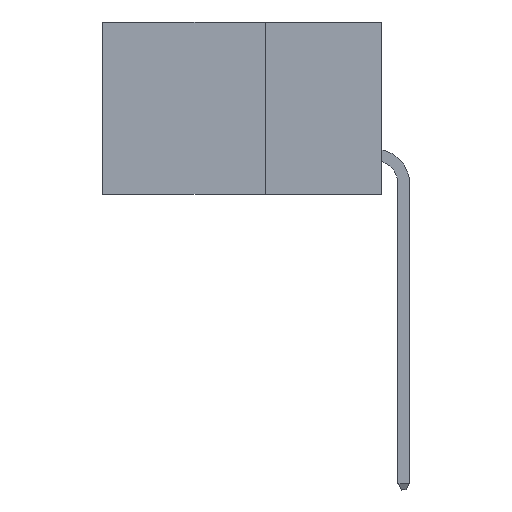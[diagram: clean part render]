
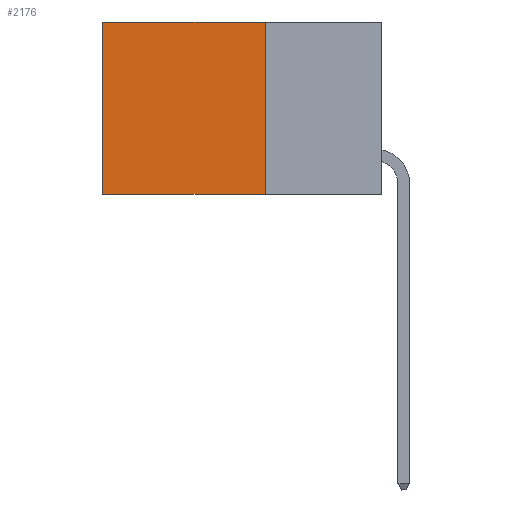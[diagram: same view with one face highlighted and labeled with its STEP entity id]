
A CAD part, left-side view. The second image highlights one B-rep face of the part: STEP entity #2176.
In plain terms, the highlighted planar face has unit normal (-1, 0, 0).
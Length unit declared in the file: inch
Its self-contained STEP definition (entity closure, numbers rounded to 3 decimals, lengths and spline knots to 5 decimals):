
#363 = CARTESIAN_POINT ( 'NONE',  ( 0.2875, 0.25, -0.37 ) ) ;
#565 = CARTESIAN_POINT ( 'NONE',  ( 0.2875, 0.6, -0.37 ) ) ;
#636 = AXIS2_PLACEMENT_3D ( 'NONE', #1433, #10157, #8273 ) ;
#751 = VECTOR ( 'NONE', #8281, 39.37008 ) ;
#756 = VERTEX_POINT ( 'NONE', #565 ) ;
#850 = ORIENTED_EDGE ( 'NONE', *, *, #8083, .T. ) ;
#936 = ORIENTED_EDGE ( 'NONE', *, *, #11797, .F. ) ;
#1433 = CARTESIAN_POINT ( 'NONE',  ( 0.2875, 0.25, 0. ) ) ;
#1704 = ORIENTED_EDGE ( 'NONE', *, *, #9207, .F. ) ;
#1867 = FACE_OUTER_BOUND ( 'NONE', #2895, .T. ) ;
#2176 = ADVANCED_FACE ( 'NONE', ( #1867 ), #11308, .F. ) ;
#2213 = CARTESIAN_POINT ( 'NONE',  ( 0.2875, 0.6, 0. ) ) ;
#2643 = VERTEX_POINT ( 'NONE', #8590 ) ;
#2895 = EDGE_LOOP ( 'NONE', ( #10967, #1704, #936, #850 ) ) ;
#3516 = CARTESIAN_POINT ( 'NONE',  ( 0.2875, 0.25, 0. ) ) ;
#3892 = LINE ( 'NONE', #10457, #9092 ) ;
#3984 = VERTEX_POINT ( 'NONE', #12282 ) ;
#4860 = LINE ( 'NONE', #3516, #10936 ) ;
#5132 = DIRECTION ( 'NONE',  ( 0., 1., 0. ) ) ;
#5669 = DIRECTION ( 'NONE',  ( 0., 0., -1. ) ) ;
#6412 = VECTOR ( 'NONE', #5132, 39.37008 ) ;
#7299 = EDGE_CURVE ( 'NONE', #2643, #756, #11234, .T. ) ;
#7333 = LINE ( 'NONE', #363, #6412 ) ;
#7717 = VERTEX_POINT ( 'NONE', #11484 ) ;
#8083 = EDGE_CURVE ( 'NONE', #7717, #2643, #3892, .T. ) ;
#8273 = DIRECTION ( 'NONE',  ( 0., 0., -1. ) ) ;
#8281 = DIRECTION ( 'NONE',  ( 0., 0., -1. ) ) ;
#8590 = CARTESIAN_POINT ( 'NONE',  ( 0.2875, 0.6, 0. ) ) ;
#9092 = VECTOR ( 'NONE', #11489, 39.37008 ) ;
#9207 = EDGE_CURVE ( 'NONE', #3984, #756, #7333, .T. ) ;
#10157 = DIRECTION ( 'NONE',  ( 1., 0., 0. ) ) ;
#10457 = CARTESIAN_POINT ( 'NONE',  ( 0.2875, 0.25, 0. ) ) ;
#10936 = VECTOR ( 'NONE', #5669, 39.37008 ) ;
#10967 = ORIENTED_EDGE ( 'NONE', *, *, #7299, .T. ) ;
#11234 = LINE ( 'NONE', #2213, #751 ) ;
#11308 = PLANE ( 'NONE',  #636 ) ;
#11484 = CARTESIAN_POINT ( 'NONE',  ( 0.2875, 0.25, 0. ) ) ;
#11489 = DIRECTION ( 'NONE',  ( 0., 1., 0. ) ) ;
#11797 = EDGE_CURVE ( 'NONE', #7717, #3984, #4860, .T. ) ;
#12282 = CARTESIAN_POINT ( 'NONE',  ( 0.2875, 0.25, -0.37 ) ) ;
